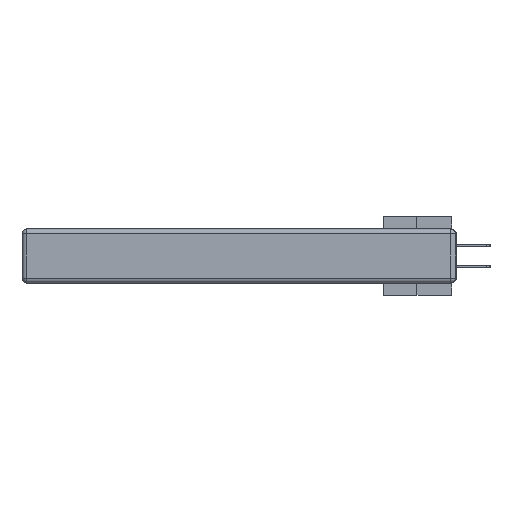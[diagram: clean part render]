
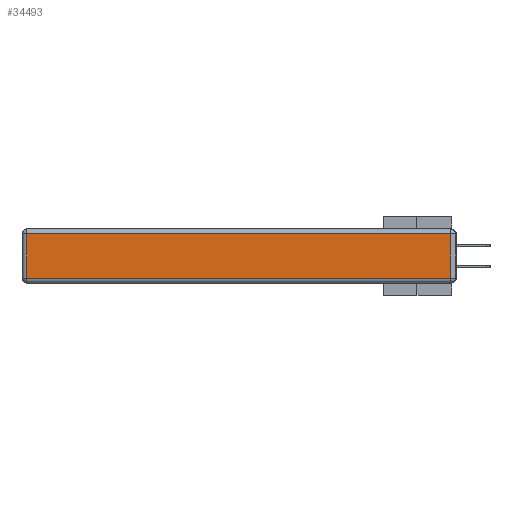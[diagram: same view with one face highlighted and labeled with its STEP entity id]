
A CAD part, left-side view. The second image highlights one B-rep face of the part: STEP entity #34493.
In plain terms, the highlighted planar face has unit normal (-1, 0, 0).
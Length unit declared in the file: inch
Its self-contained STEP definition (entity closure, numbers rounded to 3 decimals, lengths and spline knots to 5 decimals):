
#387 = VERTEX_POINT ( 'NONE', #44934 ) ;
#948 = ORIENTED_EDGE ( 'NONE', *, *, #29509, .T. ) ;
#2037 = CARTESIAN_POINT ( 'NONE',  ( 0., 2.72, -0.343 ) ) ;
#2333 = ORIENTED_EDGE ( 'NONE', *, *, #14197, .T. ) ;
#3398 = DIRECTION ( 'NONE',  ( 0., -1., 0. ) ) ;
#4209 = VERTEX_POINT ( 'NONE', #31353 ) ;
#6972 = LINE ( 'NONE', #26722, #33067 ) ;
#7703 = VERTEX_POINT ( 'NONE', #42536 ) ;
#12794 = FACE_OUTER_BOUND ( 'NONE', #18735, .T. ) ;
#13595 = LINE ( 'NONE', #40187, #42617 ) ;
#14193 = VECTOR ( 'NONE', #31711, 39.37008 ) ;
#14197 = EDGE_CURVE ( 'NONE', #7703, #39248, #6972, .T. ) ;
#16984 = ORIENTED_EDGE ( 'NONE', *, *, #27883, .T. ) ;
#17472 = LINE ( 'NONE', #37621, #25618 ) ;
#18735 = EDGE_LOOP ( 'NONE', ( #28511, #2333, #948, #16984 ) ) ;
#19161 = CARTESIAN_POINT ( 'NONE',  ( 0., 0., -0.343 ) ) ;
#22868 = DIRECTION ( 'NONE',  ( 0., 0., 1. ) ) ;
#25618 = VECTOR ( 'NONE', #39406, 39.37008 ) ;
#26722 = CARTESIAN_POINT ( 'NONE',  ( 0., 0.03, -0.343 ) ) ;
#27663 = EDGE_CURVE ( 'NONE', #387, #7703, #13595, .T. ) ;
#27883 = EDGE_CURVE ( 'NONE', #4209, #387, #47884, .T. ) ;
#28511 = ORIENTED_EDGE ( 'NONE', *, *, #27663, .T. ) ;
#29509 = EDGE_CURVE ( 'NONE', #39248, #4209, #17472, .T. ) ;
#30147 = DIRECTION ( 'NONE',  ( 0., 0., 1. ) ) ;
#30728 = CARTESIAN_POINT ( 'NONE',  ( 0., 0.03, -0.03 ) ) ;
#31353 = CARTESIAN_POINT ( 'NONE',  ( 0., 2.72, -0.03 ) ) ;
#31711 = DIRECTION ( 'NONE',  ( 0., 0., -1. ) ) ;
#33067 = VECTOR ( 'NONE', #30147, 39.37008 ) ;
#34493 = ADVANCED_FACE ( 'NONE', ( #12794 ), #41310, .T. ) ;
#37621 = CARTESIAN_POINT ( 'NONE',  ( 0., 2.75, -0.03 ) ) ;
#39248 = VERTEX_POINT ( 'NONE', #30728 ) ;
#39406 = DIRECTION ( 'NONE',  ( 0., 1., 0. ) ) ;
#39431 = AXIS2_PLACEMENT_3D ( 'NONE', #19161, #45093, #22868 ) ;
#40187 = CARTESIAN_POINT ( 'NONE',  ( 0., 0., -0.313 ) ) ;
#41310 = PLANE ( 'NONE',  #39431 ) ;
#42536 = CARTESIAN_POINT ( 'NONE',  ( 0., 0.03, -0.313 ) ) ;
#42617 = VECTOR ( 'NONE', #3398, 39.37008 ) ;
#44934 = CARTESIAN_POINT ( 'NONE',  ( 0., 2.72, -0.313 ) ) ;
#45093 = DIRECTION ( 'NONE',  ( -1., 0., 0. ) ) ;
#47884 = LINE ( 'NONE', #2037, #14193 ) ;
